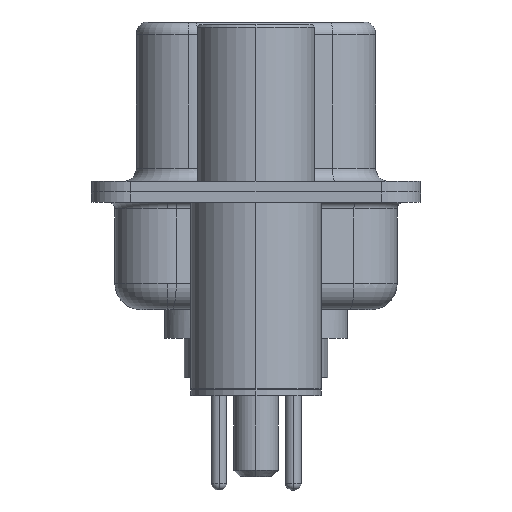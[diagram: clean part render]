
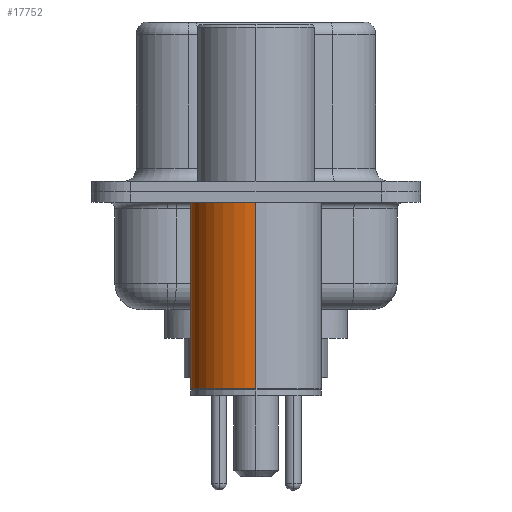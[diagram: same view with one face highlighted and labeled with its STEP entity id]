
A CAD part, left-side view. The second image highlights one B-rep face of the part: STEP entity #17752.
In plain terms, the highlighted cylindrical face has radius 2.5 mm (diameter 5 mm), a partial arc.
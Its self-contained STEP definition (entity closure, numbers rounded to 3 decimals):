
#643 = CARTESIAN_POINT ( 'NONE',  ( 0., 0., -0.4 ) ) ;
#1328 = CARTESIAN_POINT ( 'NONE',  ( -2.5, 0., 0.581 ) ) ;
#2113 = CARTESIAN_POINT ( 'NONE',  ( 2.5, 0., 0.581 ) ) ;
#2187 = DIRECTION ( 'NONE',  ( 1., 0., 0. ) ) ;
#2753 = ORIENTED_EDGE ( 'NONE', *, *, #11570, .T. ) ;
#4398 = DIRECTION ( 'NONE',  ( 0., 0., 1. ) ) ;
#5012 = LINE ( 'NONE', #1328, #12115 ) ;
#5901 = DIRECTION ( 'NONE',  ( 0., 0., 1. ) ) ;
#6162 = LINE ( 'NONE', #2113, #9234 ) ;
#6197 = AXIS2_PLACEMENT_3D ( 'NONE', #17302, #8638, #18638 ) ;
#6627 = CYLINDRICAL_SURFACE ( 'NONE', #16994, 2.5 ) ;
#7200 = CARTESIAN_POINT ( 'NONE',  ( -2.5, 0., -7.525 ) ) ;
#7467 = CARTESIAN_POINT ( 'NONE',  ( 0., 0., 0.581 ) ) ;
#8483 = AXIS2_PLACEMENT_3D ( 'NONE', #643, #11183, #2187 ) ;
#8638 = DIRECTION ( 'NONE',  ( 0., 0., 1. ) ) ;
#8729 = VERTEX_POINT ( 'NONE', #16483 ) ;
#8961 = DIRECTION ( 'NONE',  ( 1., 0., 0. ) ) ;
#9234 = VECTOR ( 'NONE', #9576, 1000. ) ;
#9463 = VERTEX_POINT ( 'NONE', #16151 ) ;
#9576 = DIRECTION ( 'NONE',  ( 0., 0., 1. ) ) ;
#11092 = FACE_OUTER_BOUND ( 'NONE', #18313, .T. ) ;
#11183 = DIRECTION ( 'NONE',  ( 0., 0., 1. ) ) ;
#11570 = EDGE_CURVE ( 'NONE', #15944, #17505, #15768, .T. ) ;
#12115 = VECTOR ( 'NONE', #4398, 1000. ) ;
#13721 = CIRCLE ( 'NONE', #8483, 2.5 ) ;
#15277 = EDGE_CURVE ( 'NONE', #15944, #8729, #6162, .T. ) ;
#15282 = EDGE_CURVE ( 'NONE', #8729, #9463, #13721, .T. ) ;
#15768 = CIRCLE ( 'NONE', #6197, 2.5 ) ;
#15777 = ORIENTED_EDGE ( 'NONE', *, *, #16011, .T. ) ;
#15944 = VERTEX_POINT ( 'NONE', #17461 ) ;
#16011 = EDGE_CURVE ( 'NONE', #17505, #9463, #5012, .T. ) ;
#16151 = CARTESIAN_POINT ( 'NONE',  ( -2.5, 0., -0.4 ) ) ;
#16483 = CARTESIAN_POINT ( 'NONE',  ( 2.5, 0., -0.4 ) ) ;
#16994 = AXIS2_PLACEMENT_3D ( 'NONE', #7467, #5901, #8961 ) ;
#17302 = CARTESIAN_POINT ( 'NONE',  ( 0., 0., -7.525 ) ) ;
#17461 = CARTESIAN_POINT ( 'NONE',  ( 2.5, 0., -7.525 ) ) ;
#17505 = VERTEX_POINT ( 'NONE', #7200 ) ;
#17752 = ADVANCED_FACE ( 'NONE', ( #11092 ), #6627, .T. ) ;
#18109 = ORIENTED_EDGE ( 'NONE', *, *, #15277, .F. ) ;
#18313 = EDGE_LOOP ( 'NONE', ( #2753, #15777, #18337, #18109 ) ) ;
#18337 = ORIENTED_EDGE ( 'NONE', *, *, #15282, .F. ) ;
#18638 = DIRECTION ( 'NONE',  ( 1., 0., 0. ) ) ;
